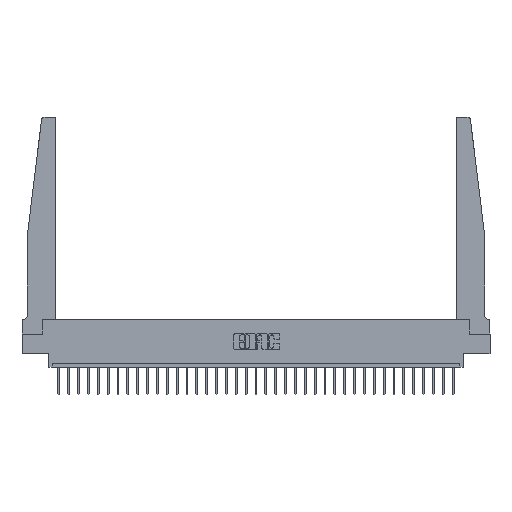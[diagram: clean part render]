
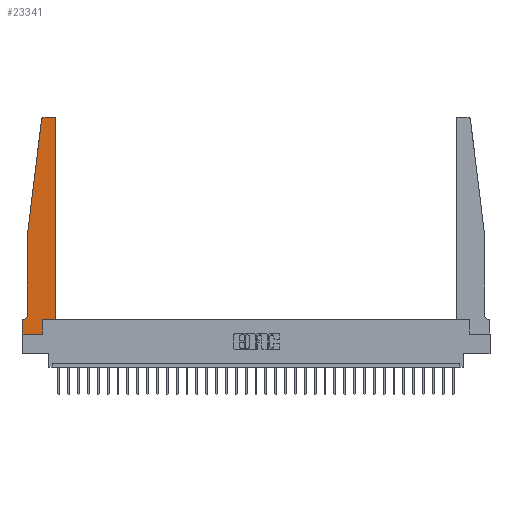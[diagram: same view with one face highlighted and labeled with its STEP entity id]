
A CAD part, top view. The second image highlights one B-rep face of the part: STEP entity #23341.
In plain terms, the highlighted planar face has unit normal (0, 0, 1).
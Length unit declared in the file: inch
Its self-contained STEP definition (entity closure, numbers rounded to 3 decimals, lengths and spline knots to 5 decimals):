
#245 = CIRCLE ( 'NONE', #17726, 0.03 ) ;
#538 = EDGE_CURVE ( 'NONE', #30414, #15072, #15313, .T. ) ;
#758 = LINE ( 'NONE', #10000, #14280 ) ;
#915 = CARTESIAN_POINT ( 'NONE',  ( 0.2605, 0.18, 0.37 ) ) ;
#1067 = ORIENTED_EDGE ( 'NONE', *, *, #26931, .T. ) ;
#2079 = DIRECTION ( 'NONE',  ( 1., 0., 0. ) ) ;
#2341 = DIRECTION ( 'NONE',  ( -1., 0., 0. ) ) ;
#3390 = CARTESIAN_POINT ( 'NONE',  ( 0.015, 0.1875, 0.37 ) ) ;
#3638 = ORIENTED_EDGE ( 'NONE', *, *, #19251, .T. ) ;
#4750 = LINE ( 'NONE', #12421, #7822 ) ;
#5120 = DIRECTION ( 'NONE',  ( 0., 0., -1. ) ) ;
#5185 = VERTEX_POINT ( 'NONE', #22813 ) ;
#5332 = ORIENTED_EDGE ( 'NONE', *, *, #538, .T. ) ;
#5460 = EDGE_CURVE ( 'NONE', #8704, #19803, #245, .T. ) ;
#5477 = EDGE_CURVE ( 'NONE', #25835, #6793, #10747, .T. ) ;
#5710 = ORIENTED_EDGE ( 'NONE', *, *, #5460, .T. ) ;
#5774 = CARTESIAN_POINT ( 'NONE',  ( 0.425, 0.18, 0.37 ) ) ;
#6092 = CARTESIAN_POINT ( 'NONE',  ( 0., 0.1875, 0.37 ) ) ;
#6214 = DIRECTION ( 'NONE',  ( 0., -1., 0. ) ) ;
#6793 = VERTEX_POINT ( 'NONE', #3390 ) ;
#6968 = ORIENTED_EDGE ( 'NONE', *, *, #25911, .T. ) ;
#7822 = VECTOR ( 'NONE', #24143, 39.37008 ) ;
#7967 = PLANE ( 'NONE',  #28725 ) ;
#8102 = DIRECTION ( 'NONE',  ( 0., 1., 0. ) ) ;
#8658 = VECTOR ( 'NONE', #2079, 39.37008 ) ;
#8704 = VERTEX_POINT ( 'NONE', #28837 ) ;
#9102 = EDGE_LOOP ( 'NONE', ( #23292, #5710, #3638, #29035, #12066, #1067, #6968, #18268, #5332, #16693, #15260, #12802 ) ) ;
#9609 = CARTESIAN_POINT ( 'NONE',  ( 0.2605, 0., 0.37 ) ) ;
#9775 = VECTOR ( 'NONE', #12706, 39.37008 ) ;
#10000 = CARTESIAN_POINT ( 'NONE',  ( 0., 0., 0.37 ) ) ;
#10107 = CARTESIAN_POINT ( 'NONE',  ( 0.395, 2.75, 0.37 ) ) ;
#10578 = EDGE_CURVE ( 'NONE', #15072, #22234, #26326, .T. ) ;
#10593 = CARTESIAN_POINT ( 'NONE',  ( 0.24675, 2.72367, 0.37 ) ) ;
#10747 = CIRCLE ( 'NONE', #24226, 0.05 ) ;
#11646 = DIRECTION ( 'NONE',  ( 0., 0., 1. ) ) ;
#12066 = ORIENTED_EDGE ( 'NONE', *, *, #5477, .T. ) ;
#12421 = CARTESIAN_POINT ( 'NONE',  ( 0.065, 0.1875, 0.37 ) ) ;
#12706 = DIRECTION ( 'NONE',  ( 0., -1., 0. ) ) ;
#12802 = ORIENTED_EDGE ( 'NONE', *, *, #16220, .T. ) ;
#13039 = VERTEX_POINT ( 'NONE', #19014 ) ;
#13404 = LINE ( 'NONE', #23092, #30746 ) ;
#13506 = CARTESIAN_POINT ( 'NONE',  ( 0.065, 1.25, 0.37 ) ) ;
#14280 = VECTOR ( 'NONE', #19207, 39.37008 ) ;
#14328 = EDGE_CURVE ( 'NONE', #13039, #25835, #13404, .T. ) ;
#14356 = CARTESIAN_POINT ( 'NONE',  ( 0.27653, 2.72, 0.37 ) ) ;
#14668 = DIRECTION ( 'NONE',  ( -1., 0., 0. ) ) ;
#15072 = VERTEX_POINT ( 'NONE', #29295 ) ;
#15215 = LINE ( 'NONE', #29753, #9775 ) ;
#15260 = ORIENTED_EDGE ( 'NONE', *, *, #28150, .T. ) ;
#15313 = LINE ( 'NONE', #915, #25395 ) ;
#15330 = FACE_OUTER_BOUND ( 'NONE', #9102, .T. ) ;
#15349 = CIRCLE ( 'NONE', #23805, 0.03 ) ;
#15386 = VECTOR ( 'NONE', #30245, 39.37008 ) ;
#15423 = EDGE_CURVE ( 'NONE', #17597, #8704, #16893, .T. ) ;
#16061 = VERTEX_POINT ( 'NONE', #20246 ) ;
#16220 = EDGE_CURVE ( 'NONE', #16061, #17597, #15349, .T. ) ;
#16462 = CARTESIAN_POINT ( 'NONE',  ( 0.425, 0.18, 0.37 ) ) ;
#16693 = ORIENTED_EDGE ( 'NONE', *, *, #10578, .T. ) ;
#16893 = LINE ( 'NONE', #26450, #29791 ) ;
#17002 = DIRECTION ( 'NONE',  ( 1., 0., 0. ) ) ;
#17597 = VERTEX_POINT ( 'NONE', #10107 ) ;
#17726 = AXIS2_PLACEMENT_3D ( 'NONE', #14356, #28444, #17002 ) ;
#18268 = ORIENTED_EDGE ( 'NONE', *, *, #26116, .T. ) ;
#19014 = CARTESIAN_POINT ( 'NONE',  ( 0.065, 1.25, 0.37 ) ) ;
#19207 = DIRECTION ( 'NONE',  ( 1., 0., 0. ) ) ;
#19251 = EDGE_CURVE ( 'NONE', #19803, #13039, #25390, .T. ) ;
#19426 = CARTESIAN_POINT ( 'NONE',  ( 0.065, 0.2375, 0.37 ) ) ;
#19803 = VERTEX_POINT ( 'NONE', #10593 ) ;
#19999 = DIRECTION ( 'NONE',  ( 1., 0., 0. ) ) ;
#20246 = CARTESIAN_POINT ( 'NONE',  ( 0.425, 2.72, 0.37 ) ) ;
#21174 = CARTESIAN_POINT ( 'NONE',  ( 0.425, 0.18, 0.37 ) ) ;
#21310 = DIRECTION ( 'NONE',  ( 1., 0., 0. ) ) ;
#22234 = VERTEX_POINT ( 'NONE', #5774 ) ;
#22813 = CARTESIAN_POINT ( 'NONE',  ( 0., 0., 0.37 ) ) ;
#23092 = CARTESIAN_POINT ( 'NONE',  ( 0.065, 1.25, 0.37 ) ) ;
#23292 = ORIENTED_EDGE ( 'NONE', *, *, #15423, .T. ) ;
#23341 = ADVANCED_FACE ( 'NONE', ( #15330 ), #7967, .T. ) ;
#23532 = LINE ( 'NONE', #21174, #26366 ) ;
#23728 = CARTESIAN_POINT ( 'NONE',  ( 0.015, 0.2375, 0.37 ) ) ;
#23805 = AXIS2_PLACEMENT_3D ( 'NONE', #28228, #11646, #21310 ) ;
#24143 = DIRECTION ( 'NONE',  ( -1., 0., 0. ) ) ;
#24226 = AXIS2_PLACEMENT_3D ( 'NONE', #23728, #5120, #14668 ) ;
#25113 = CARTESIAN_POINT ( 'NONE',  ( 0., 0.1875, 0.37 ) ) ;
#25390 = LINE ( 'NONE', #13506, #15386 ) ;
#25395 = VECTOR ( 'NONE', #8102, 39.37008 ) ;
#25835 = VERTEX_POINT ( 'NONE', #19426 ) ;
#25911 = EDGE_CURVE ( 'NONE', #27889, #5185, #15215, .T. ) ;
#26116 = EDGE_CURVE ( 'NONE', #5185, #30414, #758, .T. ) ;
#26326 = LINE ( 'NONE', #16462, #8658 ) ;
#26366 = VECTOR ( 'NONE', #30892, 39.37008 ) ;
#26450 = CARTESIAN_POINT ( 'NONE',  ( 0.25, 2.75, 0.37 ) ) ;
#26931 = EDGE_CURVE ( 'NONE', #6793, #27889, #4750, .T. ) ;
#27523 = DIRECTION ( 'NONE',  ( 0., 0., 1. ) ) ;
#27889 = VERTEX_POINT ( 'NONE', #25113 ) ;
#28150 = EDGE_CURVE ( 'NONE', #22234, #16061, #23532, .T. ) ;
#28228 = CARTESIAN_POINT ( 'NONE',  ( 0.395, 2.72, 0.37 ) ) ;
#28444 = DIRECTION ( 'NONE',  ( 0., 0., 1. ) ) ;
#28725 = AXIS2_PLACEMENT_3D ( 'NONE', #6092, #27523, #19999 ) ;
#28837 = CARTESIAN_POINT ( 'NONE',  ( 0.27653, 2.75, 0.37 ) ) ;
#29035 = ORIENTED_EDGE ( 'NONE', *, *, #14328, .T. ) ;
#29295 = CARTESIAN_POINT ( 'NONE',  ( 0.2605, 0.18, 0.37 ) ) ;
#29753 = CARTESIAN_POINT ( 'NONE',  ( 0., 0., 0.37 ) ) ;
#29791 = VECTOR ( 'NONE', #2341, 39.37008 ) ;
#30245 = DIRECTION ( 'NONE',  ( -0.122, -0.992, 0. ) ) ;
#30414 = VERTEX_POINT ( 'NONE', #9609 ) ;
#30746 = VECTOR ( 'NONE', #6214, 39.37008 ) ;
#30892 = DIRECTION ( 'NONE',  ( 0., 1., 0. ) ) ;
